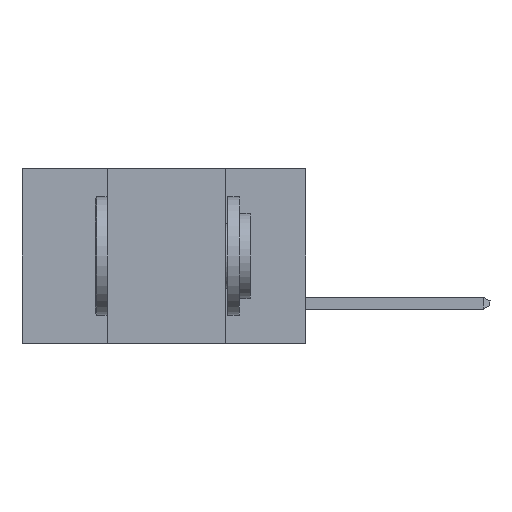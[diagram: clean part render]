
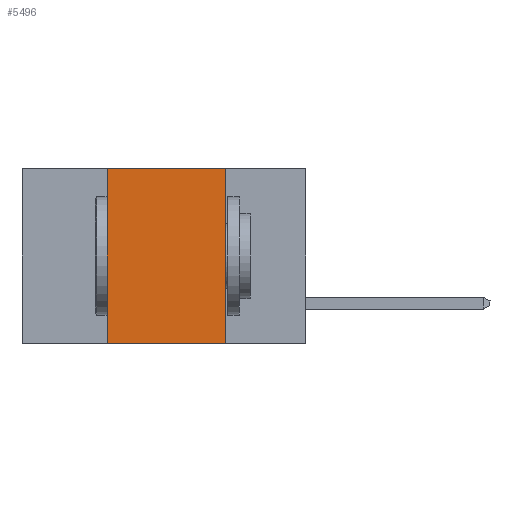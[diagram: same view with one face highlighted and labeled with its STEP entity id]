
A CAD part, left-side view. The second image highlights one B-rep face of the part: STEP entity #5496.
In plain terms, the highlighted planar face has unit normal (-1, 0, 0).
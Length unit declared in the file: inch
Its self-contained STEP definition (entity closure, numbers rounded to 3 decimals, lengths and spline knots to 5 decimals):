
#79 = CARTESIAN_POINT ( 'NONE',  ( 0., 0.6, 0. ) ) ;
#564 = AXIS2_PLACEMENT_3D ( 'NONE', #2247, #12952, #2342 ) ;
#1057 = VERTEX_POINT ( 'NONE', #12754 ) ;
#1594 = VERTEX_POINT ( 'NONE', #7411 ) ;
#2147 = CARTESIAN_POINT ( 'NONE',  ( 0., 0.17, 0. ) ) ;
#2247 = CARTESIAN_POINT ( 'NONE',  ( 0., 0.6, 0. ) ) ;
#2342 = DIRECTION ( 'NONE',  ( 0., 0., -1. ) ) ;
#2875 = VECTOR ( 'NONE', #16474, 39.37008 ) ;
#2906 = VERTEX_POINT ( 'NONE', #2147 ) ;
#3143 = CARTESIAN_POINT ( 'NONE',  ( 0., 0.6, -0.37 ) ) ;
#3172 = EDGE_LOOP ( 'NONE', ( #10991, #12554, #3536, #12794 ) ) ;
#3536 = ORIENTED_EDGE ( 'NONE', *, *, #4190, .F. ) ;
#3933 = PLANE ( 'NONE',  #564 ) ;
#4190 = EDGE_CURVE ( 'NONE', #1594, #4837, #12521, .T. ) ;
#4837 = VERTEX_POINT ( 'NONE', #13694 ) ;
#5496 = ADVANCED_FACE ( 'NONE', ( #13121 ), #3933, .F. ) ;
#6452 = EDGE_CURVE ( 'NONE', #2906, #1057, #14015, .T. ) ;
#6863 = EDGE_CURVE ( 'NONE', #1594, #1057, #15235, .T. ) ;
#7259 = CARTESIAN_POINT ( 'NONE',  ( 0., 0.42, -0.37 ) ) ;
#7411 = CARTESIAN_POINT ( 'NONE',  ( 0., 0.42, -0.37 ) ) ;
#7422 = DIRECTION ( 'NONE',  ( 0., -1., 0. ) ) ;
#8715 = VECTOR ( 'NONE', #8749, 39.37008 ) ;
#8749 = DIRECTION ( 'NONE',  ( 0., 0., 1. ) ) ;
#9374 = LINE ( 'NONE', #79, #15751 ) ;
#10991 = ORIENTED_EDGE ( 'NONE', *, *, #6452, .F. ) ;
#12521 = LINE ( 'NONE', #7259, #8715 ) ;
#12524 = DIRECTION ( 'NONE',  ( 0., -1., 0. ) ) ;
#12554 = ORIENTED_EDGE ( 'NONE', *, *, #16116, .F. ) ;
#12754 = CARTESIAN_POINT ( 'NONE',  ( 0., 0.17, -0.37 ) ) ;
#12794 = ORIENTED_EDGE ( 'NONE', *, *, #6863, .T. ) ;
#12952 = DIRECTION ( 'NONE',  ( 1., 0., 0. ) ) ;
#13121 = FACE_OUTER_BOUND ( 'NONE', #3172, .T. ) ;
#13694 = CARTESIAN_POINT ( 'NONE',  ( 0., 0.42, 0. ) ) ;
#14015 = LINE ( 'NONE', #15252, #2875 ) ;
#14065 = VECTOR ( 'NONE', #7422, 39.37008 ) ;
#15235 = LINE ( 'NONE', #3143, #14065 ) ;
#15252 = CARTESIAN_POINT ( 'NONE',  ( 0., 0.17, -0.37 ) ) ;
#15751 = VECTOR ( 'NONE', #12524, 39.37008 ) ;
#16116 = EDGE_CURVE ( 'NONE', #4837, #2906, #9374, .T. ) ;
#16474 = DIRECTION ( 'NONE',  ( 0., 0., -1. ) ) ;
